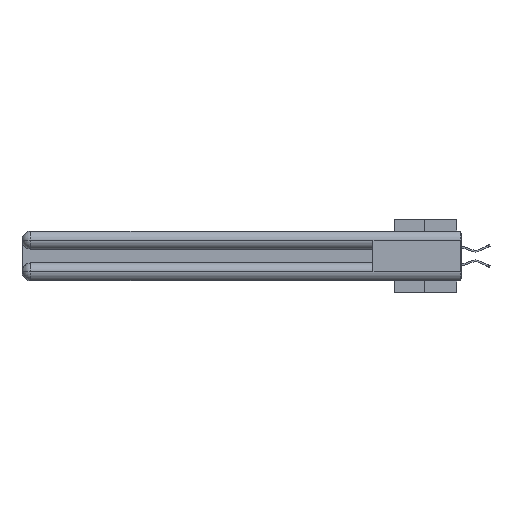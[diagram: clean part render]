
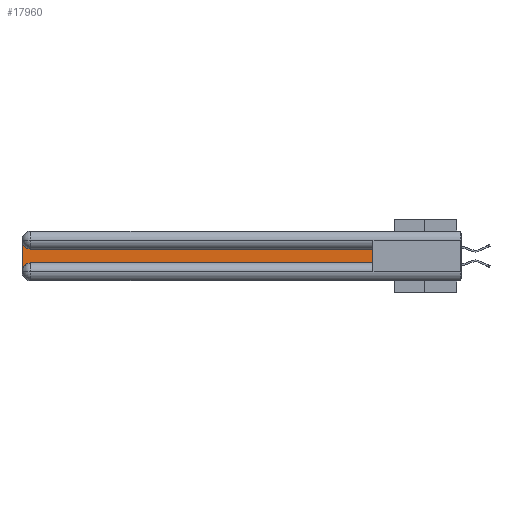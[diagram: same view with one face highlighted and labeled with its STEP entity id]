
A CAD part, left-side view. The second image highlights one B-rep face of the part: STEP entity #17960.
In plain terms, the highlighted planar face has unit normal (-1, 0, 0).
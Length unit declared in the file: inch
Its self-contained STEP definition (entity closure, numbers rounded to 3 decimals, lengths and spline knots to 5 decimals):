
#678 = ORIENTED_EDGE ( 'NONE', *, *, #18666, .T. ) ;
#1648 = VECTOR ( 'NONE', #4140, 39.37008 ) ;
#1837 = VERTEX_POINT ( 'NONE', #10307 ) ;
#2868 = VERTEX_POINT ( 'NONE', #16884 ) ;
#3195 = VECTOR ( 'NONE', #25998, 39.37008 ) ;
#4140 = DIRECTION ( 'NONE',  ( 0., 1., 0. ) ) ;
#4573 = CARTESIAN_POINT ( 'NONE',  ( 0.075, 0.6, -0.1225 ) ) ;
#4955 = CIRCLE ( 'NONE', #5687, 0.06 ) ;
#5299 = DIRECTION ( 'NONE',  ( 0., 0., -1. ) ) ;
#5486 = VECTOR ( 'NONE', #19332, 39.37008 ) ;
#5687 = AXIS2_PLACEMENT_3D ( 'NONE', #14876, #27828, #5299 ) ;
#6120 = EDGE_CURVE ( 'NONE', #28786, #42272, #11369, .T. ) ;
#6437 = CARTESIAN_POINT ( 'NONE',  ( 0.075, 0.6, -0.2175 ) ) ;
#6650 = EDGE_LOOP ( 'NONE', ( #37737, #11663, #678, #41149, #38758, #28476 ) ) ;
#9345 = EDGE_CURVE ( 'NONE', #2868, #11106, #20179, .T. ) ;
#10307 = CARTESIAN_POINT ( 'NONE',  ( 0.075, 3., -0.0625 ) ) ;
#10742 = AXIS2_PLACEMENT_3D ( 'NONE', #22461, #25332, #35254 ) ;
#11106 = VERTEX_POINT ( 'NONE', #41645 ) ;
#11281 = CARTESIAN_POINT ( 'NONE',  ( 0.075, 2.94, -0.2775 ) ) ;
#11369 = CIRCLE ( 'NONE', #33738, 0.06 ) ;
#11414 = CARTESIAN_POINT ( 'NONE',  ( 0.075, 2.94, -0.1225 ) ) ;
#11663 = ORIENTED_EDGE ( 'NONE', *, *, #32779, .T. ) ;
#14876 = CARTESIAN_POINT ( 'NONE',  ( 0.075, 2.94, -0.0625 ) ) ;
#15686 = PLANE ( 'NONE',  #10742 ) ;
#16884 = CARTESIAN_POINT ( 'NONE',  ( 0.075, 0.6, -0.2175 ) ) ;
#17015 = EDGE_CURVE ( 'NONE', #42272, #2868, #22958, .T. ) ;
#17127 = CARTESIAN_POINT ( 'NONE',  ( 0.075, 2.94, -0.2175 ) ) ;
#17960 = ADVANCED_FACE ( 'NONE', ( #41627 ), #15686, .F. ) ;
#18666 = EDGE_CURVE ( 'NONE', #1837, #28786, #26818, .T. ) ;
#19020 = EDGE_CURVE ( 'NONE', #11106, #22370, #29412, .T. ) ;
#19332 = DIRECTION ( 'NONE',  ( 0., -1., 0. ) ) ;
#20179 = LINE ( 'NONE', #30162, #37679 ) ;
#22370 = VERTEX_POINT ( 'NONE', #11414 ) ;
#22461 = CARTESIAN_POINT ( 'NONE',  ( 0.075, 3., -0.1225 ) ) ;
#22958 = LINE ( 'NONE', #6437, #5486 ) ;
#24182 = DIRECTION ( 'NONE',  ( 0., 0., -1. ) ) ;
#24482 = CARTESIAN_POINT ( 'NONE',  ( 0.075, 3., -0.2775 ) ) ;
#25332 = DIRECTION ( 'NONE',  ( 1., 0., 0. ) ) ;
#25998 = DIRECTION ( 'NONE',  ( 0., 0., -1. ) ) ;
#26818 = LINE ( 'NONE', #29175, #3195 ) ;
#27238 = DIRECTION ( 'NONE',  ( 0., 0., 1. ) ) ;
#27828 = DIRECTION ( 'NONE',  ( 1., 0., 0. ) ) ;
#28074 = DIRECTION ( 'NONE',  ( 1., 0., 0. ) ) ;
#28476 = ORIENTED_EDGE ( 'NONE', *, *, #9345, .T. ) ;
#28786 = VERTEX_POINT ( 'NONE', #24482 ) ;
#29175 = CARTESIAN_POINT ( 'NONE',  ( 0.075, 3., -0.2175 ) ) ;
#29412 = LINE ( 'NONE', #4573, #1648 ) ;
#30162 = CARTESIAN_POINT ( 'NONE',  ( 0.075, 0.6, -0.2175 ) ) ;
#32779 = EDGE_CURVE ( 'NONE', #22370, #1837, #4955, .T. ) ;
#33738 = AXIS2_PLACEMENT_3D ( 'NONE', #11281, #28074, #24182 ) ;
#35254 = DIRECTION ( 'NONE',  ( 0., 0., -1. ) ) ;
#37679 = VECTOR ( 'NONE', #27238, 39.37008 ) ;
#37737 = ORIENTED_EDGE ( 'NONE', *, *, #19020, .T. ) ;
#38758 = ORIENTED_EDGE ( 'NONE', *, *, #17015, .T. ) ;
#41149 = ORIENTED_EDGE ( 'NONE', *, *, #6120, .T. ) ;
#41627 = FACE_OUTER_BOUND ( 'NONE', #6650, .T. ) ;
#41645 = CARTESIAN_POINT ( 'NONE',  ( 0.075, 0.6, -0.1225 ) ) ;
#42272 = VERTEX_POINT ( 'NONE', #17127 ) ;
